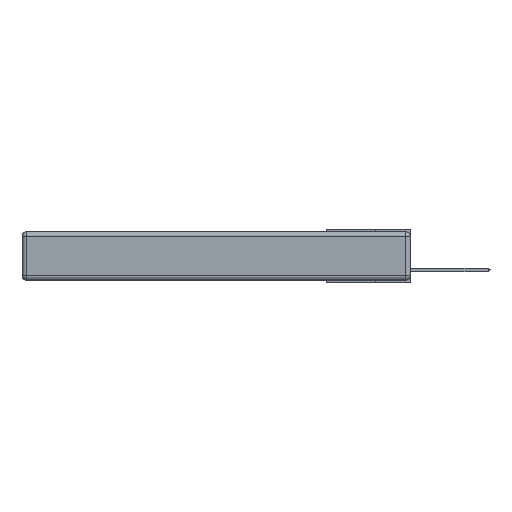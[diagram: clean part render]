
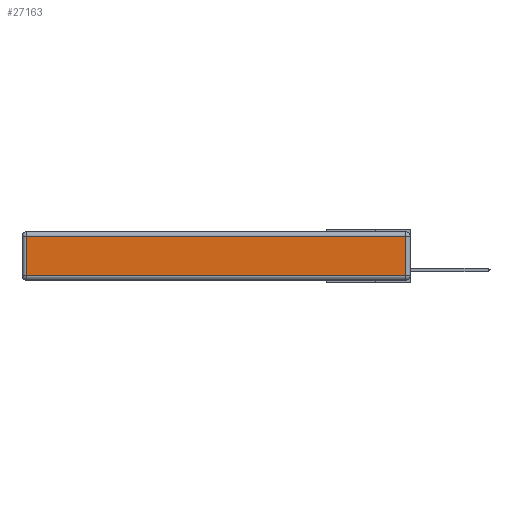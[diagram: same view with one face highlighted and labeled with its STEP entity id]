
A CAD part, left-side view. The second image highlights one B-rep face of the part: STEP entity #27163.
In plain terms, the highlighted planar face has unit normal (-1, 0, 0).
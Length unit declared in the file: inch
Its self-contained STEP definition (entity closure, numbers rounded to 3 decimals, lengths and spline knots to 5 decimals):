
#241 = ORIENTED_EDGE ( 'NONE', *, *, #7601, .T. ) ;
#602 = LINE ( 'NONE', #1478, #12081 ) ;
#1153 = VECTOR ( 'NONE', #18961, 39.37008 ) ;
#1478 = CARTESIAN_POINT ( 'NONE',  ( 0., 0., -0.313 ) ) ;
#1872 = CARTESIAN_POINT ( 'NONE',  ( 0., 2.72, -0.03 ) ) ;
#2549 = DIRECTION ( 'NONE',  ( 0., -1., 0. ) ) ;
#2765 = EDGE_CURVE ( 'NONE', #12234, #21048, #602, .T. ) ;
#2928 = CARTESIAN_POINT ( 'NONE',  ( 0., 0.03, -0.343 ) ) ;
#3309 = DIRECTION ( 'NONE',  ( -1., 0., 0. ) ) ;
#3655 = ORIENTED_EDGE ( 'NONE', *, *, #22534, .T. ) ;
#5460 = DIRECTION ( 'NONE',  ( 0., 1., 0. ) ) ;
#6070 = LINE ( 'NONE', #14348, #7512 ) ;
#6129 = ORIENTED_EDGE ( 'NONE', *, *, #2765, .T. ) ;
#6172 = CARTESIAN_POINT ( 'NONE',  ( 0., 0.03, -0.03 ) ) ;
#7472 = DIRECTION ( 'NONE',  ( 0., 0., -1. ) ) ;
#7512 = VECTOR ( 'NONE', #5460, 39.37008 ) ;
#7601 = EDGE_CURVE ( 'NONE', #21048, #11286, #10878, .T. ) ;
#8170 = FACE_OUTER_BOUND ( 'NONE', #28186, .T. ) ;
#9213 = VECTOR ( 'NONE', #7472, 39.37008 ) ;
#10878 = LINE ( 'NONE', #2928, #1153 ) ;
#11286 = VERTEX_POINT ( 'NONE', #6172 ) ;
#12081 = VECTOR ( 'NONE', #2549, 39.37008 ) ;
#12234 = VERTEX_POINT ( 'NONE', #21242 ) ;
#13020 = EDGE_CURVE ( 'NONE', #20910, #12234, #21786, .T. ) ;
#13547 = CARTESIAN_POINT ( 'NONE',  ( 0., 0.03, -0.313 ) ) ;
#14348 = CARTESIAN_POINT ( 'NONE',  ( 0., 2.75, -0.03 ) ) ;
#18961 = DIRECTION ( 'NONE',  ( 0., 0., 1. ) ) ;
#19444 = PLANE ( 'NONE',  #28583 ) ;
#20910 = VERTEX_POINT ( 'NONE', #1872 ) ;
#21048 = VERTEX_POINT ( 'NONE', #13547 ) ;
#21242 = CARTESIAN_POINT ( 'NONE',  ( 0., 2.72, -0.313 ) ) ;
#21786 = LINE ( 'NONE', #25724, #9213 ) ;
#22534 = EDGE_CURVE ( 'NONE', #11286, #20910, #6070, .T. ) ;
#23776 = CARTESIAN_POINT ( 'NONE',  ( 0., 0., -0.343 ) ) ;
#25723 = ORIENTED_EDGE ( 'NONE', *, *, #13020, .T. ) ;
#25724 = CARTESIAN_POINT ( 'NONE',  ( 0., 2.72, -0.343 ) ) ;
#27163 = ADVANCED_FACE ( 'NONE', ( #8170 ), #19444, .T. ) ;
#28186 = EDGE_LOOP ( 'NONE', ( #6129, #241, #3655, #25723 ) ) ;
#28379 = DIRECTION ( 'NONE',  ( 0., 0., 1. ) ) ;
#28583 = AXIS2_PLACEMENT_3D ( 'NONE', #23776, #3309, #28379 ) ;
